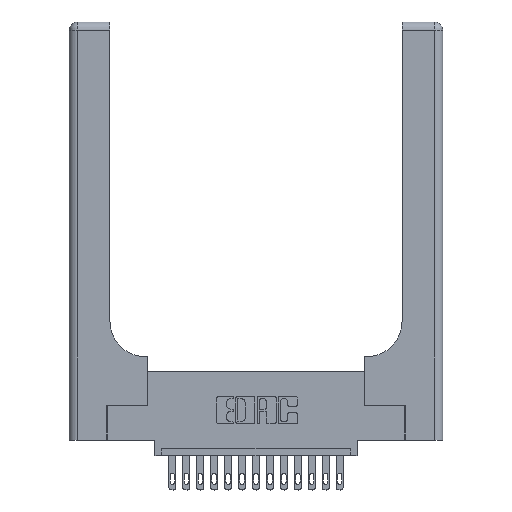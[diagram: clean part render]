
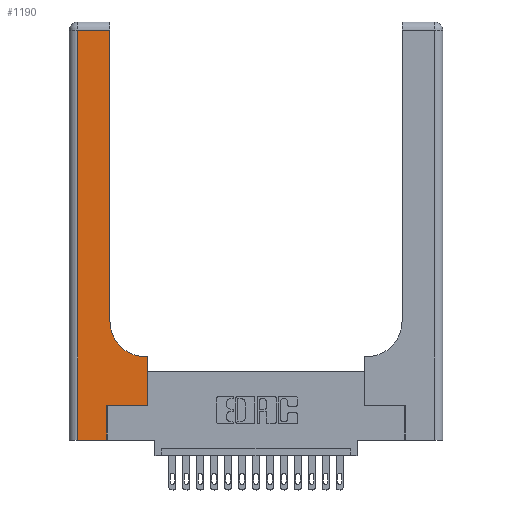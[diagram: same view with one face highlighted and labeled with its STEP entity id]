
A CAD part, top view. The second image highlights one B-rep face of the part: STEP entity #1190.
In plain terms, the highlighted planar face has unit normal (0, 0, 1).
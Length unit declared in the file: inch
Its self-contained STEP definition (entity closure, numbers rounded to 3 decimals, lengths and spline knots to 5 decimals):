
#113 = CARTESIAN_POINT ( 'NONE',  ( 0.269, 0.25, 0.37 ) ) ;
#654 = ORIENTED_EDGE ( 'NONE', *, *, #8573, .T. ) ;
#1026 = VECTOR ( 'NONE', #14483, 39.37008 ) ;
#1190 = ADVANCED_FACE ( 'NONE', ( #12610 ), #4982, .F. ) ;
#1255 = CARTESIAN_POINT ( 'NONE',  ( 0.269, 0., 0.37 ) ) ;
#1618 = CARTESIAN_POINT ( 'NONE',  ( 0.2915, 0.6, 0.37 ) ) ;
#2355 = AXIS2_PLACEMENT_3D ( 'NONE', #3553, #18249, #6630 ) ;
#2561 = AXIS2_PLACEMENT_3D ( 'NONE', #15458, #16917, #15572 ) ;
#2600 = ORIENTED_EDGE ( 'NONE', *, *, #14761, .T. ) ;
#2934 = CARTESIAN_POINT ( 'NONE',  ( 0., 2.94, 0.37 ) ) ;
#3181 = DIRECTION ( 'NONE',  ( -1., 0., 0. ) ) ;
#3425 = ORIENTED_EDGE ( 'NONE', *, *, #7776, .T. ) ;
#3493 = CARTESIAN_POINT ( 'NONE',  ( 0.06, 2.94, 0.37 ) ) ;
#3553 = CARTESIAN_POINT ( 'NONE',  ( 0., 3., 0.37 ) ) ;
#3748 = CARTESIAN_POINT ( 'NONE',  ( 0.269, 0.25, 0.37 ) ) ;
#3826 = EDGE_CURVE ( 'NONE', #4630, #8237, #4275, .T. ) ;
#3930 = LINE ( 'NONE', #1618, #13543 ) ;
#4275 = LINE ( 'NONE', #7221, #17534 ) ;
#4630 = VERTEX_POINT ( 'NONE', #3493 ) ;
#4669 = VERTEX_POINT ( 'NONE', #3748 ) ;
#4810 = VECTOR ( 'NONE', #10728, 39.37008 ) ;
#4982 = PLANE ( 'NONE',  #2355 ) ;
#5143 = CARTESIAN_POINT ( 'NONE',  ( 0.2915, 2.94, 0.37 ) ) ;
#5967 = LINE ( 'NONE', #8098, #18526 ) ;
#6041 = ORIENTED_EDGE ( 'NONE', *, *, #9116, .T. ) ;
#6276 = ORIENTED_EDGE ( 'NONE', *, *, #9269, .T. ) ;
#6630 = DIRECTION ( 'NONE',  ( -1., 0., 0. ) ) ;
#6637 = EDGE_CURVE ( 'NONE', #4669, #9425, #12694, .T. ) ;
#7221 = CARTESIAN_POINT ( 'NONE',  ( 0.06, 3., 0.37 ) ) ;
#7488 = DIRECTION ( 'NONE',  ( -1., 0., 0. ) ) ;
#7776 = EDGE_CURVE ( 'NONE', #10241, #18628, #3930, .T. ) ;
#7844 = VERTEX_POINT ( 'NONE', #11031 ) ;
#8076 = VERTEX_POINT ( 'NONE', #1255 ) ;
#8098 = CARTESIAN_POINT ( 'NONE',  ( 0., 0., 0.37 ) ) ;
#8237 = VERTEX_POINT ( 'NONE', #8840 ) ;
#8273 = VECTOR ( 'NONE', #3181, 39.37008 ) ;
#8573 = EDGE_CURVE ( 'NONE', #9425, #10241, #17651, .T. ) ;
#8840 = CARTESIAN_POINT ( 'NONE',  ( 0.06, 0., 0.37 ) ) ;
#9116 = EDGE_CURVE ( 'NONE', #18140, #4630, #13754, .T. ) ;
#9269 = EDGE_CURVE ( 'NONE', #8076, #4669, #9875, .T. ) ;
#9367 = EDGE_CURVE ( 'NONE', #18628, #7844, #17846, .T. ) ;
#9425 = VERTEX_POINT ( 'NONE', #11138 ) ;
#9875 = LINE ( 'NONE', #13463, #4810 ) ;
#10241 = VERTEX_POINT ( 'NONE', #15675 ) ;
#10594 = EDGE_LOOP ( 'NONE', ( #12490, #6041, #11381, #2600, #6276, #17283, #654, #3425, #13351 ) ) ;
#10728 = DIRECTION ( 'NONE',  ( 0., 1., 0. ) ) ;
#11031 = CARTESIAN_POINT ( 'NONE',  ( 0.2915, 0.85, 0.37 ) ) ;
#11138 = CARTESIAN_POINT ( 'NONE',  ( 0.5585, 0.25, 0.37 ) ) ;
#11381 = ORIENTED_EDGE ( 'NONE', *, *, #3826, .T. ) ;
#11516 = DIRECTION ( 'NONE',  ( 0., 1., 0. ) ) ;
#11607 = LINE ( 'NONE', #17235, #13411 ) ;
#12414 = VECTOR ( 'NONE', #17053, 39.37008 ) ;
#12490 = ORIENTED_EDGE ( 'NONE', *, *, #17132, .T. ) ;
#12610 = FACE_OUTER_BOUND ( 'NONE', #10594, .T. ) ;
#12694 = LINE ( 'NONE', #113, #1026 ) ;
#13299 = DIRECTION ( 'NONE',  ( 0., -1., 0. ) ) ;
#13351 = ORIENTED_EDGE ( 'NONE', *, *, #9367, .T. ) ;
#13411 = VECTOR ( 'NONE', #11516, 39.37008 ) ;
#13463 = CARTESIAN_POINT ( 'NONE',  ( 0.269, 0., 0.37 ) ) ;
#13543 = VECTOR ( 'NONE', #7488, 39.37008 ) ;
#13754 = LINE ( 'NONE', #2934, #8273 ) ;
#13968 = DIRECTION ( 'NONE',  ( 1., 0., 0. ) ) ;
#14074 = CARTESIAN_POINT ( 'NONE',  ( 0.5415, 0.6, 0.37 ) ) ;
#14483 = DIRECTION ( 'NONE',  ( 1., 0., 0. ) ) ;
#14761 = EDGE_CURVE ( 'NONE', #8237, #8076, #5967, .T. ) ;
#15458 = CARTESIAN_POINT ( 'NONE',  ( 0.5415, 0.85, 0.37 ) ) ;
#15572 = DIRECTION ( 'NONE',  ( 1., 0., 0. ) ) ;
#15675 = CARTESIAN_POINT ( 'NONE',  ( 0.5585, 0.6, 0.37 ) ) ;
#16917 = DIRECTION ( 'NONE',  ( 0., 0., -1. ) ) ;
#16987 = CARTESIAN_POINT ( 'NONE',  ( 0.5585, 0.25, 0.37 ) ) ;
#17053 = DIRECTION ( 'NONE',  ( 0., 1., 0. ) ) ;
#17132 = EDGE_CURVE ( 'NONE', #7844, #18140, #11607, .T. ) ;
#17235 = CARTESIAN_POINT ( 'NONE',  ( 0.2915, 3., 0.37 ) ) ;
#17283 = ORIENTED_EDGE ( 'NONE', *, *, #6637, .T. ) ;
#17534 = VECTOR ( 'NONE', #13299, 39.37008 ) ;
#17651 = LINE ( 'NONE', #16987, #12414 ) ;
#17846 = CIRCLE ( 'NONE', #2561, 0.25 ) ;
#18140 = VERTEX_POINT ( 'NONE', #5143 ) ;
#18249 = DIRECTION ( 'NONE',  ( 0., 0., -1. ) ) ;
#18526 = VECTOR ( 'NONE', #13968, 39.37008 ) ;
#18628 = VERTEX_POINT ( 'NONE', #14074 ) ;
